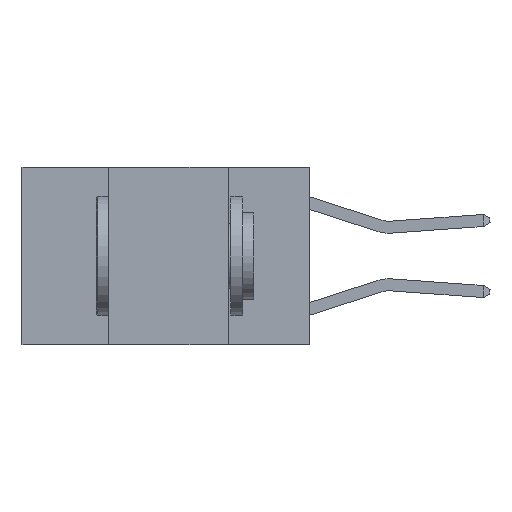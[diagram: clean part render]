
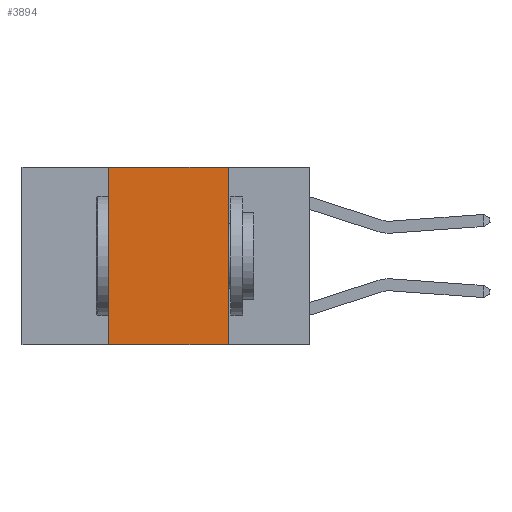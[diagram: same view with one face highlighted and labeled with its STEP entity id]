
A CAD part, left-side view. The second image highlights one B-rep face of the part: STEP entity #3894.
In plain terms, the highlighted planar face has unit normal (-1, 0, 0).
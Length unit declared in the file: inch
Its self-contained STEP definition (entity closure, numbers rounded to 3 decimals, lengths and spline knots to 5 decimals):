
#810 = ORIENTED_EDGE ( 'NONE', *, *, #16407, .F. ) ;
#1979 = LINE ( 'NONE', #16512, #17019 ) ;
#2389 = EDGE_CURVE ( 'NONE', #7754, #10362, #7621, .T. ) ;
#3351 = PLANE ( 'NONE',  #7372 ) ;
#3894 = ADVANCED_FACE ( 'NONE', ( #7622 ), #3351, .F. ) ;
#4525 = DIRECTION ( 'NONE',  ( 0., -1., 0. ) ) ;
#5393 = VECTOR ( 'NONE', #22486, 39.37008 ) ;
#7036 = ORIENTED_EDGE ( 'NONE', *, *, #14603, .F. ) ;
#7055 = VECTOR ( 'NONE', #4525, 39.37008 ) ;
#7372 = AXIS2_PLACEMENT_3D ( 'NONE', #14455, #10636, #21707 ) ;
#7530 = CARTESIAN_POINT ( 'NONE',  ( 0., 0.17, 0. ) ) ;
#7621 = LINE ( 'NONE', #22134, #5393 ) ;
#7622 = FACE_OUTER_BOUND ( 'NONE', #21520, .T. ) ;
#7754 = VERTEX_POINT ( 'NONE', #7530 ) ;
#9017 = ORIENTED_EDGE ( 'NONE', *, *, #2389, .F. ) ;
#10362 = VERTEX_POINT ( 'NONE', #16081 ) ;
#10489 = VERTEX_POINT ( 'NONE', #22122 ) ;
#10636 = DIRECTION ( 'NONE',  ( 1., 0., 0. ) ) ;
#11013 = VECTOR ( 'NONE', #11700, 39.37008 ) ;
#11700 = DIRECTION ( 'NONE',  ( 0., -1., 0. ) ) ;
#12961 = EDGE_CURVE ( 'NONE', #22709, #10362, #21064, .T. ) ;
#14148 = CARTESIAN_POINT ( 'NONE',  ( 0., 0.6, -0.37 ) ) ;
#14455 = CARTESIAN_POINT ( 'NONE',  ( 0., 0.6, 0. ) ) ;
#14603 = EDGE_CURVE ( 'NONE', #22709, #10489, #1979, .T. ) ;
#14974 = ORIENTED_EDGE ( 'NONE', *, *, #12961, .T. ) ;
#15298 = LINE ( 'NONE', #22561, #11013 ) ;
#16081 = CARTESIAN_POINT ( 'NONE',  ( 0., 0.17, -0.37 ) ) ;
#16407 = EDGE_CURVE ( 'NONE', #10489, #7754, #15298, .T. ) ;
#16512 = CARTESIAN_POINT ( 'NONE',  ( 0., 0.42, 0. ) ) ;
#16985 = DIRECTION ( 'NONE',  ( 0., 0., 1. ) ) ;
#17019 = VECTOR ( 'NONE', #16985, 39.37008 ) ;
#20488 = CARTESIAN_POINT ( 'NONE',  ( 0., 0.42, -0.37 ) ) ;
#21064 = LINE ( 'NONE', #14148, #7055 ) ;
#21520 = EDGE_LOOP ( 'NONE', ( #9017, #810, #7036, #14974 ) ) ;
#21707 = DIRECTION ( 'NONE',  ( 0., 0., -1. ) ) ;
#22122 = CARTESIAN_POINT ( 'NONE',  ( 0., 0.42, 0. ) ) ;
#22134 = CARTESIAN_POINT ( 'NONE',  ( 0., 0.17, 0. ) ) ;
#22486 = DIRECTION ( 'NONE',  ( 0., 0., -1. ) ) ;
#22561 = CARTESIAN_POINT ( 'NONE',  ( 0., 0.6, 0. ) ) ;
#22709 = VERTEX_POINT ( 'NONE', #20488 ) ;
